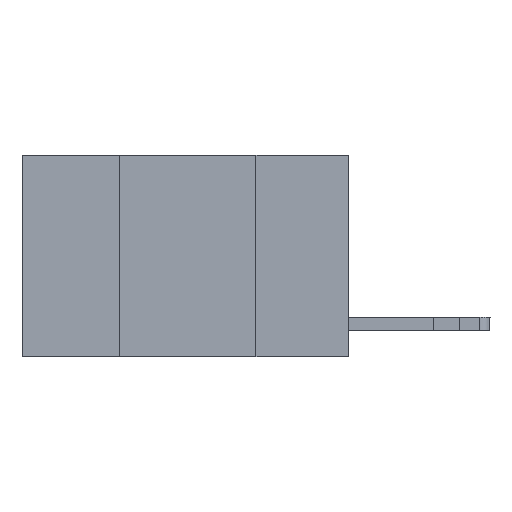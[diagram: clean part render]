
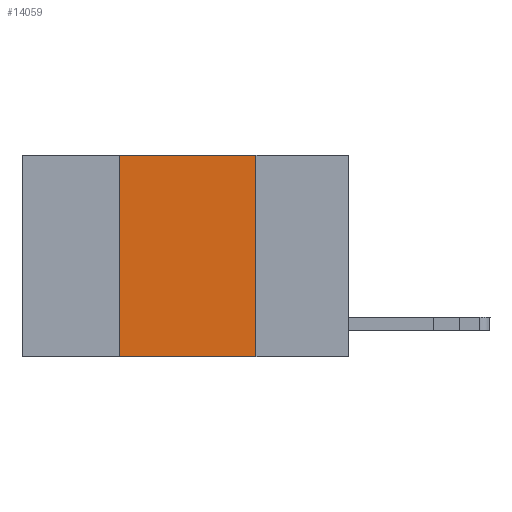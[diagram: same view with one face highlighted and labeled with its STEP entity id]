
A CAD part, left-side view. The second image highlights one B-rep face of the part: STEP entity #14059.
In plain terms, the highlighted planar face has unit normal (-1, 0, 0).
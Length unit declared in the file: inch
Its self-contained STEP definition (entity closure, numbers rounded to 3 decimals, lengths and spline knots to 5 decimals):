
#78 = VERTEX_POINT ( 'NONE', #10341 ) ;
#392 = ORIENTED_EDGE ( 'NONE', *, *, #7180, .F. ) ;
#1258 = EDGE_CURVE ( 'NONE', #3092, #78, #3212, .T. ) ;
#1813 = AXIS2_PLACEMENT_3D ( 'NONE', #14406, #15837, #7635 ) ;
#2578 = VERTEX_POINT ( 'NONE', #15410 ) ;
#2870 = DIRECTION ( 'NONE',  ( 0., 0., -1. ) ) ;
#3092 = VERTEX_POINT ( 'NONE', #15279 ) ;
#3212 = LINE ( 'NONE', #15147, #17423 ) ;
#3321 = CARTESIAN_POINT ( 'NONE',  ( 0., 0.42, 0. ) ) ;
#3774 = EDGE_LOOP ( 'NONE', ( #16987, #6478, #392, #14997 ) ) ;
#4961 = VERTEX_POINT ( 'NONE', #3321 ) ;
#5146 = CARTESIAN_POINT ( 'NONE',  ( 0., 0.6, 0. ) ) ;
#5494 = CARTESIAN_POINT ( 'NONE',  ( 0., 0.42, 0. ) ) ;
#6478 = ORIENTED_EDGE ( 'NONE', *, *, #15916, .F. ) ;
#7180 = EDGE_CURVE ( 'NONE', #2578, #4961, #7709, .T. ) ;
#7635 = DIRECTION ( 'NONE',  ( 0., 0., -1. ) ) ;
#7709 = LINE ( 'NONE', #5494, #10431 ) ;
#7900 = CARTESIAN_POINT ( 'NONE',  ( 0., 0.6, -0.37 ) ) ;
#9046 = VECTOR ( 'NONE', #17544, 39.37008 ) ;
#9552 = DIRECTION ( 'NONE',  ( 0., 0., 1. ) ) ;
#10126 = FACE_OUTER_BOUND ( 'NONE', #3774, .T. ) ;
#10341 = CARTESIAN_POINT ( 'NONE',  ( 0., 0.17, -0.37 ) ) ;
#10431 = VECTOR ( 'NONE', #9552, 39.37008 ) ;
#12969 = PLANE ( 'NONE',  #1813 ) ;
#14059 = ADVANCED_FACE ( 'NONE', ( #10126 ), #12969, .F. ) ;
#14406 = CARTESIAN_POINT ( 'NONE',  ( 0., 0.6, 0. ) ) ;
#14745 = LINE ( 'NONE', #5146, #15632 ) ;
#14815 = EDGE_CURVE ( 'NONE', #2578, #78, #15933, .T. ) ;
#14997 = ORIENTED_EDGE ( 'NONE', *, *, #14815, .T. ) ;
#15147 = CARTESIAN_POINT ( 'NONE',  ( 0., 0.17, 0. ) ) ;
#15279 = CARTESIAN_POINT ( 'NONE',  ( 0., 0.17, 0. ) ) ;
#15410 = CARTESIAN_POINT ( 'NONE',  ( 0., 0.42, -0.37 ) ) ;
#15632 = VECTOR ( 'NONE', #16091, 39.37008 ) ;
#15837 = DIRECTION ( 'NONE',  ( 1., 0., 0. ) ) ;
#15916 = EDGE_CURVE ( 'NONE', #4961, #3092, #14745, .T. ) ;
#15933 = LINE ( 'NONE', #7900, #9046 ) ;
#16091 = DIRECTION ( 'NONE',  ( 0., -1., 0. ) ) ;
#16987 = ORIENTED_EDGE ( 'NONE', *, *, #1258, .F. ) ;
#17423 = VECTOR ( 'NONE', #2870, 39.37008 ) ;
#17544 = DIRECTION ( 'NONE',  ( 0., -1., 0. ) ) ;
